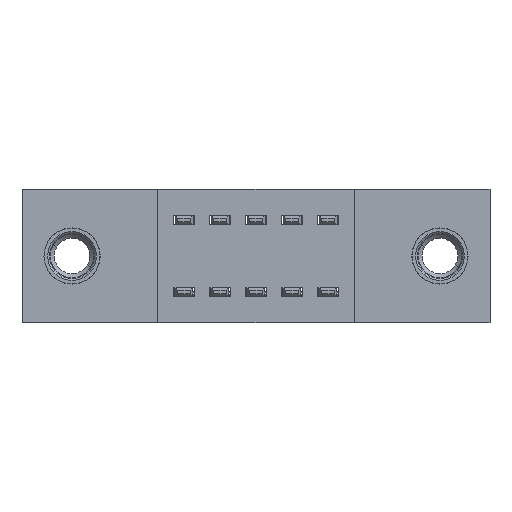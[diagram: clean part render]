
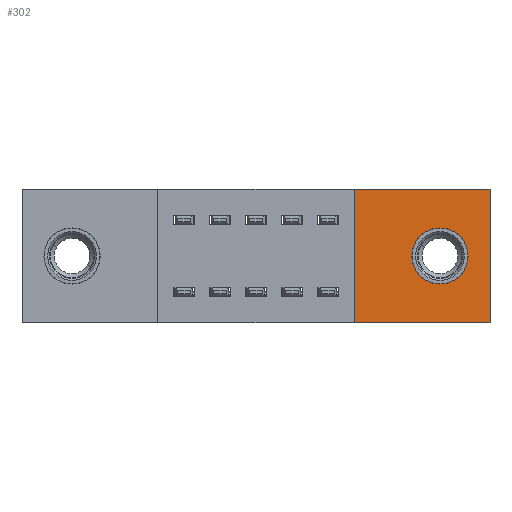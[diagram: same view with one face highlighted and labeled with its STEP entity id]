
A CAD part, front view. The second image highlights one B-rep face of the part: STEP entity #302.
In plain terms, the highlighted planar face has unit normal (0, -1, 0).
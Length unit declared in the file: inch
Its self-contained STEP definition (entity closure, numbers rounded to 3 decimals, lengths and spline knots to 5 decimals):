
#186 = VERTEX_POINT ( 'NONE', #2741 ) ;
#266 = CARTESIAN_POINT ( 'NONE',  ( 1.161, 0., -0.107 ) ) ;
#302 = ADVANCED_FACE ( 'NONE', ( #2268, #7856 ), #4340, .T. ) ;
#646 = AXIS2_PLACEMENT_3D ( 'NONE', #2606, #5563, #5797 ) ;
#994 = CARTESIAN_POINT ( 'NONE',  ( 1.3, 0., -0.37 ) ) ;
#1004 = ORIENTED_EDGE ( 'NONE', *, *, #8122, .F. ) ;
#1132 = CARTESIAN_POINT ( 'NONE',  ( 0.923, 0., 0. ) ) ;
#1429 = CARTESIAN_POINT ( 'NONE',  ( 1.3, 0., 0. ) ) ;
#1448 = AXIS2_PLACEMENT_3D ( 'NONE', #4298, #6094, #6422 ) ;
#1450 = EDGE_CURVE ( 'NONE', #186, #4552, #2139, .T. ) ;
#1752 = CARTESIAN_POINT ( 'NONE',  ( 1.3, 0., 0. ) ) ;
#1777 = LINE ( 'NONE', #7704, #8307 ) ;
#1887 = EDGE_CURVE ( 'NONE', #7922, #5661, #7573, .T. ) ;
#1983 = ORIENTED_EDGE ( 'NONE', *, *, #3416, .F. ) ;
#2139 = CIRCLE ( 'NONE', #646, 0.078 ) ;
#2268 = FACE_BOUND ( 'NONE', #8332, .T. ) ;
#2296 = EDGE_CURVE ( 'NONE', #4552, #186, #8598, .T. ) ;
#2461 = DIRECTION ( 'NONE',  ( 0., 0., -1. ) ) ;
#2474 = EDGE_CURVE ( 'NONE', #5661, #3708, #5567, .T. ) ;
#2606 = CARTESIAN_POINT ( 'NONE',  ( 1.161, 0., -0.185 ) ) ;
#2741 = CARTESIAN_POINT ( 'NONE',  ( 1.161, 0., -0.263 ) ) ;
#2824 = DIRECTION ( 'NONE',  ( 0., 1., 0. ) ) ;
#2938 = CARTESIAN_POINT ( 'NONE',  ( 0., 0., -0.37 ) ) ;
#3416 = EDGE_CURVE ( 'NONE', #3708, #6636, #6813, .T. ) ;
#3708 = VERTEX_POINT ( 'NONE', #5050 ) ;
#3718 = DIRECTION ( 'NONE',  ( 1., 0., 0. ) ) ;
#3817 = EDGE_LOOP ( 'NONE', ( #1983, #6308, #4734, #1004 ) ) ;
#4298 = CARTESIAN_POINT ( 'NONE',  ( 0., 0., -0.37 ) ) ;
#4340 = PLANE ( 'NONE',  #1448 ) ;
#4458 = AXIS2_PLACEMENT_3D ( 'NONE', #6826, #2824, #7502 ) ;
#4552 = VERTEX_POINT ( 'NONE', #266 ) ;
#4734 = ORIENTED_EDGE ( 'NONE', *, *, #1887, .F. ) ;
#5050 = CARTESIAN_POINT ( 'NONE',  ( 0.923, 0., -0.37 ) ) ;
#5563 = DIRECTION ( 'NONE',  ( 0., 1., 0. ) ) ;
#5567 = LINE ( 'NONE', #2938, #7769 ) ;
#5661 = VERTEX_POINT ( 'NONE', #994 ) ;
#5787 = VECTOR ( 'NONE', #2461, 39.37008 ) ;
#5797 = DIRECTION ( 'NONE',  ( 0., 0., -1. ) ) ;
#6094 = DIRECTION ( 'NONE',  ( 0., -1., 0. ) ) ;
#6109 = CARTESIAN_POINT ( 'NONE',  ( 0.923, 0., -0.37 ) ) ;
#6308 = ORIENTED_EDGE ( 'NONE', *, *, #2474, .F. ) ;
#6422 = DIRECTION ( 'NONE',  ( 0., 0., -1. ) ) ;
#6636 = VERTEX_POINT ( 'NONE', #1132 ) ;
#6778 = DIRECTION ( 'NONE',  ( 0., 0., 1. ) ) ;
#6813 = LINE ( 'NONE', #6109, #8378 ) ;
#6826 = CARTESIAN_POINT ( 'NONE',  ( 1.161, 0., -0.185 ) ) ;
#6941 = DIRECTION ( 'NONE',  ( -1., 0., 0. ) ) ;
#7502 = DIRECTION ( 'NONE',  ( 0., 0., -1. ) ) ;
#7573 = LINE ( 'NONE', #1752, #5787 ) ;
#7704 = CARTESIAN_POINT ( 'NONE',  ( 0., 0., 0. ) ) ;
#7769 = VECTOR ( 'NONE', #6941, 39.37008 ) ;
#7856 = FACE_OUTER_BOUND ( 'NONE', #3817, .T. ) ;
#7922 = VERTEX_POINT ( 'NONE', #1429 ) ;
#8009 = ORIENTED_EDGE ( 'NONE', *, *, #1450, .T. ) ;
#8026 = ORIENTED_EDGE ( 'NONE', *, *, #2296, .T. ) ;
#8122 = EDGE_CURVE ( 'NONE', #6636, #7922, #1777, .T. ) ;
#8307 = VECTOR ( 'NONE', #3718, 39.37008 ) ;
#8332 = EDGE_LOOP ( 'NONE', ( #8026, #8009 ) ) ;
#8378 = VECTOR ( 'NONE', #6778, 39.37008 ) ;
#8598 = CIRCLE ( 'NONE', #4458, 0.078 ) ;
